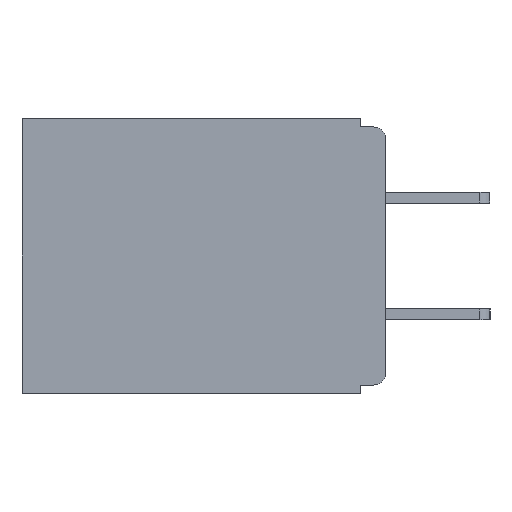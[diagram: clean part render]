
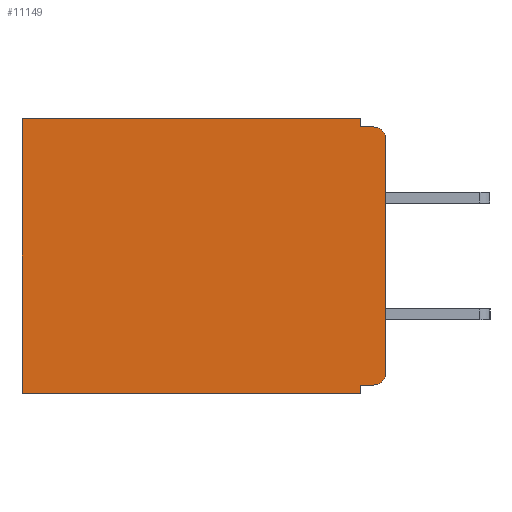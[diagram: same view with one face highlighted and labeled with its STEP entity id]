
A CAD part, left-side view. The second image highlights one B-rep face of the part: STEP entity #11149.
In plain terms, the highlighted planar face has unit normal (-1, 0, 0).
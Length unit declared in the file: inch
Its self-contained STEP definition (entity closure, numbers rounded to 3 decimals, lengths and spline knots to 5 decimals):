
#388 = EDGE_CURVE ( 'NONE', #3846, #1351, #920, .T. ) ;
#468 = DIRECTION ( 'NONE',  ( -1., 0., 0. ) ) ;
#525 = ORIENTED_EDGE ( 'NONE', *, *, #15785, .F. ) ;
#578 = VERTEX_POINT ( 'NONE', #8000 ) ;
#707 = EDGE_CURVE ( 'NONE', #9075, #12020, #9704, .T. ) ;
#711 = CARTESIAN_POINT ( 'NONE',  ( 0.3, 0., -0.025 ) ) ;
#920 = LINE ( 'NONE', #14367, #13845 ) ;
#1112 = LINE ( 'NONE', #4873, #4198 ) ;
#1351 = VERTEX_POINT ( 'NONE', #4504 ) ;
#1948 = VECTOR ( 'NONE', #10906, 39.37008 ) ;
#1963 = CARTESIAN_POINT ( 'NONE',  ( 0.3, 0.437, -0.33 ) ) ;
#1973 = ORIENTED_EDGE ( 'NONE', *, *, #3212, .T. ) ;
#2007 = CARTESIAN_POINT ( 'NONE',  ( 0.3, 0., -0.33 ) ) ;
#2266 = VERTEX_POINT ( 'NONE', #5879 ) ;
#2992 = CARTESIAN_POINT ( 'NONE',  ( 0.3, 0.437, -0.33 ) ) ;
#3114 = ORIENTED_EDGE ( 'NONE', *, *, #707, .T. ) ;
#3175 = CARTESIAN_POINT ( 'NONE',  ( 0.3, 0., -0.32 ) ) ;
#3212 = EDGE_CURVE ( 'NONE', #11285, #578, #14130, .T. ) ;
#3562 = DIRECTION ( 'NONE',  ( 0., -1., 0. ) ) ;
#3846 = VERTEX_POINT ( 'NONE', #8477 ) ;
#4045 = DIRECTION ( 'NONE',  ( 0., 0., -1. ) ) ;
#4048 = ORIENTED_EDGE ( 'NONE', *, *, #15227, .F. ) ;
#4051 = VERTEX_POINT ( 'NONE', #13804 ) ;
#4198 = VECTOR ( 'NONE', #3562, 39.37008 ) ;
#4365 = ORIENTED_EDGE ( 'NONE', *, *, #9213, .T. ) ;
#4485 = DIRECTION ( 'NONE',  ( 0., 1., 0. ) ) ;
#4499 = ORIENTED_EDGE ( 'NONE', *, *, #8217, .F. ) ;
#4504 = CARTESIAN_POINT ( 'NONE',  ( 0.3, 0.031, -0.01 ) ) ;
#4873 = CARTESIAN_POINT ( 'NONE',  ( 0.3, 0., -0.01 ) ) ;
#4907 = AXIS2_PLACEMENT_3D ( 'NONE', #5286, #13851, #6548 ) ;
#4984 = ORIENTED_EDGE ( 'NONE', *, *, #388, .F. ) ;
#5286 = CARTESIAN_POINT ( 'NONE',  ( 0.3, 0., -0.33 ) ) ;
#5879 = CARTESIAN_POINT ( 'NONE',  ( 0.3, 0.031, -0.33 ) ) ;
#5897 = DIRECTION ( 'NONE',  ( 0., 1., 0. ) ) ;
#5913 = CARTESIAN_POINT ( 'NONE',  ( 0.3, 0.031, -0.33 ) ) ;
#6421 = LINE ( 'NONE', #3175, #12578 ) ;
#6424 = FACE_OUTER_BOUND ( 'NONE', #15890, .T. ) ;
#6548 = DIRECTION ( 'NONE',  ( 0., 0., -1. ) ) ;
#6749 = VECTOR ( 'NONE', #7520, 39.37008 ) ;
#6755 = ORIENTED_EDGE ( 'NONE', *, *, #7876, .T. ) ;
#7520 = DIRECTION ( 'NONE',  ( 0., 0., -1. ) ) ;
#7682 = LINE ( 'NONE', #9004, #13619 ) ;
#7876 = EDGE_CURVE ( 'NONE', #3846, #9075, #7682, .T. ) ;
#7903 = CARTESIAN_POINT ( 'NONE',  ( 0.3, 0.437, 0. ) ) ;
#8000 = CARTESIAN_POINT ( 'NONE',  ( 0.3, 0., -0.305 ) ) ;
#8172 = CARTESIAN_POINT ( 'NONE',  ( 0.3, 0.015, -0.025 ) ) ;
#8217 = EDGE_CURVE ( 'NONE', #14155, #578, #10038, .T. ) ;
#8470 = ORIENTED_EDGE ( 'NONE', *, *, #15320, .F. ) ;
#8477 = CARTESIAN_POINT ( 'NONE',  ( 0.3, 0.031, 0. ) ) ;
#8781 = ORIENTED_EDGE ( 'NONE', *, *, #13759, .F. ) ;
#9004 = CARTESIAN_POINT ( 'NONE',  ( 0.3, 0., 0. ) ) ;
#9062 = DIRECTION ( 'NONE',  ( 0., 1., 0. ) ) ;
#9075 = VERTEX_POINT ( 'NONE', #7903 ) ;
#9213 = EDGE_CURVE ( 'NONE', #14155, #15349, #15216, .T. ) ;
#9423 = DIRECTION ( 'NONE',  ( 0., 0., -1. ) ) ;
#9704 = LINE ( 'NONE', #2992, #10082 ) ;
#9941 = CARTESIAN_POINT ( 'NONE',  ( 0.3, 0.015, -0.01 ) ) ;
#10038 = LINE ( 'NONE', #15943, #6749 ) ;
#10082 = VECTOR ( 'NONE', #4045, 39.37008 ) ;
#10906 = DIRECTION ( 'NONE',  ( 0., 0., -1. ) ) ;
#11149 = ADVANCED_FACE ( 'NONE', ( #6424 ), #11455, .F. ) ;
#11285 = VERTEX_POINT ( 'NONE', #15266 ) ;
#11386 = DIRECTION ( 'NONE',  ( -1., 0., 0. ) ) ;
#11455 = PLANE ( 'NONE',  #4907 ) ;
#11624 = AXIS2_PLACEMENT_3D ( 'NONE', #11935, #11386, #12558 ) ;
#11935 = CARTESIAN_POINT ( 'NONE',  ( 0.3, 0.015, -0.305 ) ) ;
#12020 = VERTEX_POINT ( 'NONE', #1963 ) ;
#12558 = DIRECTION ( 'NONE',  ( 0., 0., -1. ) ) ;
#12578 = VECTOR ( 'NONE', #4485, 39.37008 ) ;
#13252 = LINE ( 'NONE', #2007, #15610 ) ;
#13613 = AXIS2_PLACEMENT_3D ( 'NONE', #8172, #468, #9423 ) ;
#13619 = VECTOR ( 'NONE', #9062, 39.37008 ) ;
#13759 = EDGE_CURVE ( 'NONE', #11285, #4051, #6421, .T. ) ;
#13804 = CARTESIAN_POINT ( 'NONE',  ( 0.3, 0.031, -0.32 ) ) ;
#13845 = VECTOR ( 'NONE', #14842, 39.37008 ) ;
#13851 = DIRECTION ( 'NONE',  ( 1., 0., 0. ) ) ;
#14130 = CIRCLE ( 'NONE', #11624, 0.015 ) ;
#14155 = VERTEX_POINT ( 'NONE', #711 ) ;
#14367 = CARTESIAN_POINT ( 'NONE',  ( 0.3, 0.031, 0. ) ) ;
#14842 = DIRECTION ( 'NONE',  ( 0., 0., -1. ) ) ;
#15095 = LINE ( 'NONE', #5913, #1948 ) ;
#15216 = CIRCLE ( 'NONE', #13613, 0.015 ) ;
#15227 = EDGE_CURVE ( 'NONE', #4051, #2266, #15095, .T. ) ;
#15266 = CARTESIAN_POINT ( 'NONE',  ( 0.3, 0.015, -0.32 ) ) ;
#15320 = EDGE_CURVE ( 'NONE', #1351, #15349, #1112, .T. ) ;
#15349 = VERTEX_POINT ( 'NONE', #9941 ) ;
#15610 = VECTOR ( 'NONE', #5897, 39.37008 ) ;
#15785 = EDGE_CURVE ( 'NONE', #2266, #12020, #13252, .T. ) ;
#15890 = EDGE_LOOP ( 'NONE', ( #4499, #4365, #8470, #4984, #6755, #3114, #525, #4048, #8781, #1973 ) ) ;
#15943 = CARTESIAN_POINT ( 'NONE',  ( 0.3, 0., -0.33 ) ) ;
